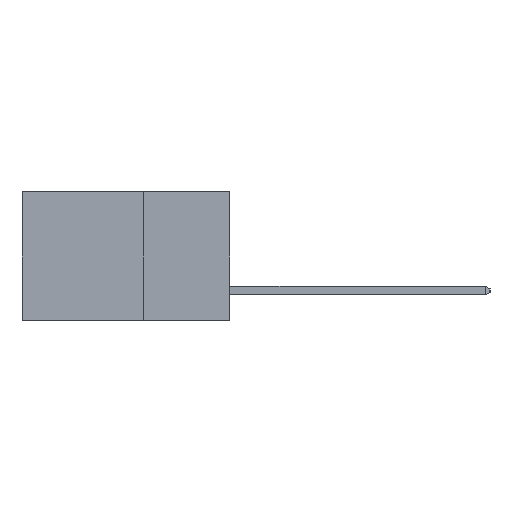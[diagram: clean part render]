
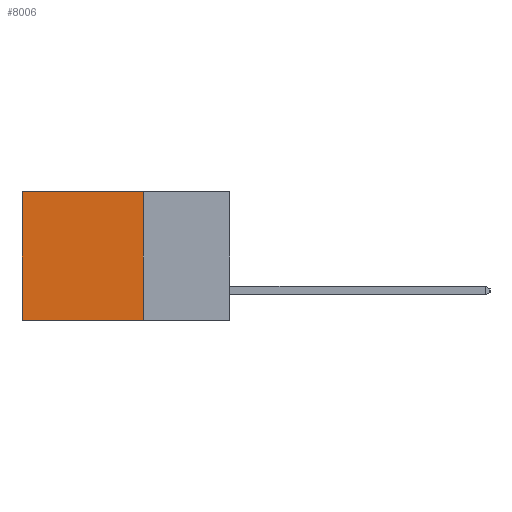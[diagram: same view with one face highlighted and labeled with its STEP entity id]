
A CAD part, left-side view. The second image highlights one B-rep face of the part: STEP entity #8006.
In plain terms, the highlighted planar face has unit normal (-1, 0, 0).
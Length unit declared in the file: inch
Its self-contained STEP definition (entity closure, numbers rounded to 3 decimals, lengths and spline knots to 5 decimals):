
#685 = LINE ( 'NONE', #5240, #8939 ) ;
#1003 = ORIENTED_EDGE ( 'NONE', *, *, #18994, .T. ) ;
#2078 = ORIENTED_EDGE ( 'NONE', *, *, #14132, .T. ) ;
#2386 = VERTEX_POINT ( 'NONE', #6058 ) ;
#2785 = EDGE_LOOP ( 'NONE', ( #2078, #11468, #18936, #1003 ) ) ;
#3554 = DIRECTION ( 'NONE',  ( 0., 0., -1. ) ) ;
#3834 = VERTEX_POINT ( 'NONE', #13684 ) ;
#4147 = CARTESIAN_POINT ( 'NONE',  ( 0.2615, 0.6, 0. ) ) ;
#4531 = DIRECTION ( 'NONE',  ( 0., 1., 0. ) ) ;
#5240 = CARTESIAN_POINT ( 'NONE',  ( 0.2615, 0.6, -0.37 ) ) ;
#5429 = VERTEX_POINT ( 'NONE', #10977 ) ;
#5578 = EDGE_CURVE ( 'NONE', #3834, #5429, #19423, .T. ) ;
#5637 = DIRECTION ( 'NONE',  ( 0., 0., -1. ) ) ;
#5701 = CARTESIAN_POINT ( 'NONE',  ( 0.2615, 0.25, -0.37 ) ) ;
#6054 = EDGE_CURVE ( 'NONE', #2386, #3834, #10931, .T. ) ;
#6058 = CARTESIAN_POINT ( 'NONE',  ( 0.2615, 0.25, 0. ) ) ;
#8006 = ADVANCED_FACE ( 'NONE', ( #16101 ), #17094, .F. ) ;
#8288 = LINE ( 'NONE', #14152, #16228 ) ;
#8939 = VECTOR ( 'NONE', #3554, 39.37008 ) ;
#9612 = DIRECTION ( 'NONE',  ( 0., 1., 0. ) ) ;
#9737 = CARTESIAN_POINT ( 'NONE',  ( 0.2615, 0.25, -0.37 ) ) ;
#10931 = LINE ( 'NONE', #5701, #14716 ) ;
#10977 = CARTESIAN_POINT ( 'NONE',  ( 0.2615, 0.6, -0.37 ) ) ;
#11468 = ORIENTED_EDGE ( 'NONE', *, *, #5578, .F. ) ;
#13684 = CARTESIAN_POINT ( 'NONE',  ( 0.2615, 0.25, -0.37 ) ) ;
#14132 = EDGE_CURVE ( 'NONE', #16807, #5429, #685, .T. ) ;
#14152 = CARTESIAN_POINT ( 'NONE',  ( 0.2615, 0.25, 0. ) ) ;
#14249 = AXIS2_PLACEMENT_3D ( 'NONE', #16769, #16580, #16502 ) ;
#14716 = VECTOR ( 'NONE', #5637, 39.37008 ) ;
#15225 = VECTOR ( 'NONE', #9612, 39.37008 ) ;
#16101 = FACE_OUTER_BOUND ( 'NONE', #2785, .T. ) ;
#16228 = VECTOR ( 'NONE', #4531, 39.37008 ) ;
#16502 = DIRECTION ( 'NONE',  ( 0., 0., -1. ) ) ;
#16580 = DIRECTION ( 'NONE',  ( 1., 0., 0. ) ) ;
#16769 = CARTESIAN_POINT ( 'NONE',  ( 0.2615, 0.25, -0.37 ) ) ;
#16807 = VERTEX_POINT ( 'NONE', #4147 ) ;
#17094 = PLANE ( 'NONE',  #14249 ) ;
#18936 = ORIENTED_EDGE ( 'NONE', *, *, #6054, .F. ) ;
#18994 = EDGE_CURVE ( 'NONE', #2386, #16807, #8288, .T. ) ;
#19423 = LINE ( 'NONE', #9737, #15225 ) ;
